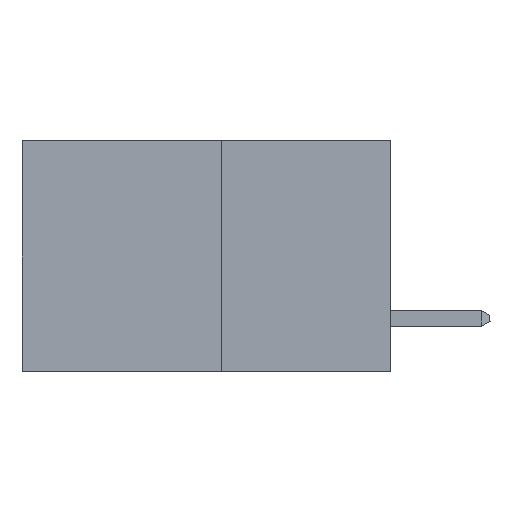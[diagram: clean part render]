
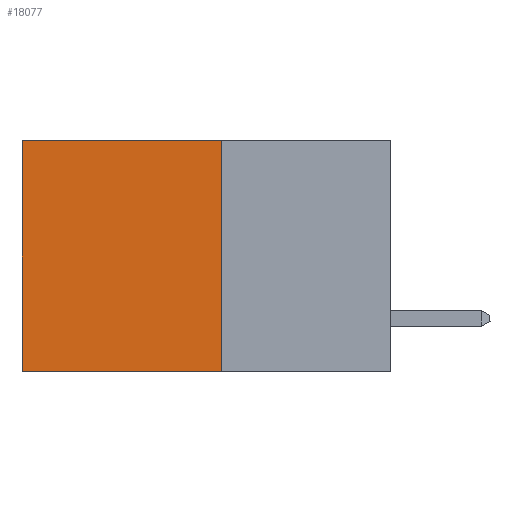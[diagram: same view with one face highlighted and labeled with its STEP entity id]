
A CAD part, left-side view. The second image highlights one B-rep face of the part: STEP entity #18077.
In plain terms, the highlighted planar face has unit normal (-1, 0, 0).
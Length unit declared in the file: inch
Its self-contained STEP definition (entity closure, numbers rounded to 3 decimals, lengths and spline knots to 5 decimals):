
#979 = PLANE ( 'NONE',  #25684 ) ;
#1547 = LINE ( 'NONE', #18192, #14343 ) ;
#1933 = CARTESIAN_POINT ( 'NONE',  ( 0.277, 0.59, -0.37 ) ) ;
#2118 = VERTEX_POINT ( 'NONE', #33001 ) ;
#2187 = DIRECTION ( 'NONE',  ( 0., 1., 0. ) ) ;
#2507 = VECTOR ( 'NONE', #5110, 39.37008 ) ;
#2517 = CARTESIAN_POINT ( 'NONE',  ( 0.277, 0.27, -0.37 ) ) ;
#3130 = ORIENTED_EDGE ( 'NONE', *, *, #19102, .F. ) ;
#3317 = LINE ( 'NONE', #20437, #2507 ) ;
#3594 = CARTESIAN_POINT ( 'NONE',  ( 0.277, 0.27, -0.37 ) ) ;
#4421 = EDGE_CURVE ( 'NONE', #2118, #22110, #21327, .T. ) ;
#5110 = DIRECTION ( 'NONE',  ( 0., 0., -1. ) ) ;
#6018 = CARTESIAN_POINT ( 'NONE',  ( 0.277, 0.59, 0. ) ) ;
#6173 = DIRECTION ( 'NONE',  ( 1., 0., 0. ) ) ;
#7428 = FACE_OUTER_BOUND ( 'NONE', #21253, .T. ) ;
#7880 = EDGE_CURVE ( 'NONE', #19947, #28198, #1547, .T. ) ;
#9828 = LINE ( 'NONE', #1933, #15747 ) ;
#12119 = DIRECTION ( 'NONE',  ( 0., 0., -1. ) ) ;
#14085 = ORIENTED_EDGE ( 'NONE', *, *, #4421, .F. ) ;
#14343 = VECTOR ( 'NONE', #18081, 39.37008 ) ;
#14448 = VECTOR ( 'NONE', #2187, 39.37008 ) ;
#15747 = VECTOR ( 'NONE', #12119, 39.37008 ) ;
#16113 = ORIENTED_EDGE ( 'NONE', *, *, #24119, .T. ) ;
#18077 = ADVANCED_FACE ( 'NONE', ( #7428 ), #979, .F. ) ;
#18081 = DIRECTION ( 'NONE',  ( 0., 1., 0. ) ) ;
#18192 = CARTESIAN_POINT ( 'NONE',  ( 0.277, 0.27, 0. ) ) ;
#19102 = EDGE_CURVE ( 'NONE', #19947, #2118, #3317, .T. ) ;
#19947 = VERTEX_POINT ( 'NONE', #29236 ) ;
#20437 = CARTESIAN_POINT ( 'NONE',  ( 0.277, 0.27, -0.37 ) ) ;
#21253 = EDGE_LOOP ( 'NONE', ( #16113, #14085, #3130, #31993 ) ) ;
#21327 = LINE ( 'NONE', #2517, #14448 ) ;
#22110 = VERTEX_POINT ( 'NONE', #25095 ) ;
#24057 = DIRECTION ( 'NONE',  ( 0., 0., -1. ) ) ;
#24119 = EDGE_CURVE ( 'NONE', #28198, #22110, #9828, .T. ) ;
#25095 = CARTESIAN_POINT ( 'NONE',  ( 0.277, 0.59, -0.37 ) ) ;
#25684 = AXIS2_PLACEMENT_3D ( 'NONE', #3594, #6173, #24057 ) ;
#28198 = VERTEX_POINT ( 'NONE', #6018 ) ;
#29236 = CARTESIAN_POINT ( 'NONE',  ( 0.277, 0.27, 0. ) ) ;
#31993 = ORIENTED_EDGE ( 'NONE', *, *, #7880, .T. ) ;
#33001 = CARTESIAN_POINT ( 'NONE',  ( 0.277, 0.27, -0.37 ) ) ;
